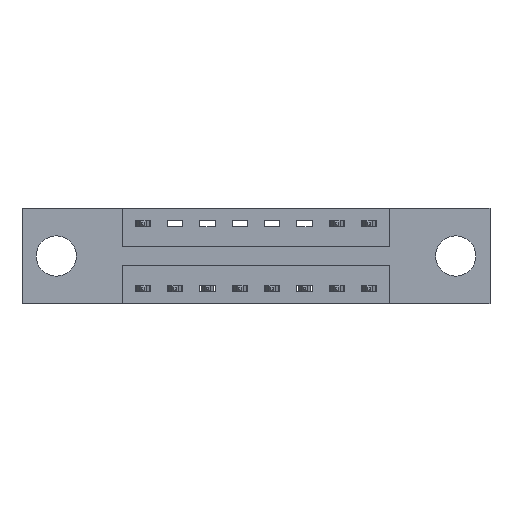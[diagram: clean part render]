
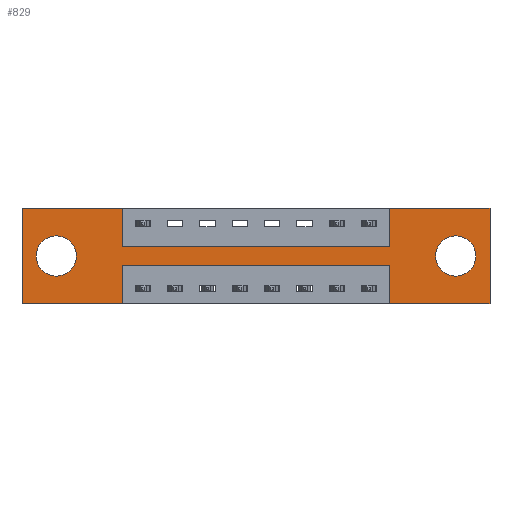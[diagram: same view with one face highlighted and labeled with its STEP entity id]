
A CAD part, front view. The second image highlights one B-rep face of the part: STEP entity #829.
In plain terms, the highlighted planar face has unit normal (0, -1, 0).
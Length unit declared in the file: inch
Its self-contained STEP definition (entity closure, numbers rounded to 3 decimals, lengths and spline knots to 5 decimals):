
#142 = AXIS2_PLACEMENT_3D ( 'NONE', #3195, #8237, #3962 ) ;
#279 = VERTEX_POINT ( 'NONE', #336 ) ;
#292 = VECTOR ( 'NONE', #1090, 39.37008 ) ;
#336 = CARTESIAN_POINT ( 'NONE',  ( 0.1325, 0., -0.107 ) ) ;
#423 = ORIENTED_EDGE ( 'NONE', *, *, #8382, .T. ) ;
#425 = ORIENTED_EDGE ( 'NONE', *, *, #6639, .T. ) ;
#449 = ORIENTED_EDGE ( 'NONE', *, *, #6753, .T. ) ;
#463 = ORIENTED_EDGE ( 'NONE', *, *, #4237, .T. ) ;
#499 = ORIENTED_EDGE ( 'NONE', *, *, #6702, .F. ) ;
#525 = ORIENTED_EDGE ( 'NONE', *, *, #2740, .F. ) ;
#550 = CARTESIAN_POINT ( 'NONE',  ( 0.1325, 0., -0.263 ) ) ;
#573 = VERTEX_POINT ( 'NONE', #4162 ) ;
#583 = EDGE_CURVE ( 'NONE', #5346, #4613, #7836, .T. ) ;
#586 = EDGE_CURVE ( 'NONE', #573, #3477, #4030, .T. ) ;
#593 = ORIENTED_EDGE ( 'NONE', *, *, #5875, .F. ) ;
#601 = VECTOR ( 'NONE', #5198, 39.37008 ) ;
#605 = ORIENTED_EDGE ( 'NONE', *, *, #6371, .F. ) ;
#628 = ORIENTED_EDGE ( 'NONE', *, *, #583, .F. ) ;
#641 = ORIENTED_EDGE ( 'NONE', *, *, #2733, .F. ) ;
#718 = ORIENTED_EDGE ( 'NONE', *, *, #4485, .F. ) ;
#726 = ORIENTED_EDGE ( 'NONE', *, *, #7225, .F. ) ;
#733 = DIRECTION ( 'NONE',  ( -1., 0., 0. ) ) ;
#740 = ORIENTED_EDGE ( 'NONE', *, *, #7984, .F. ) ;
#758 = ORIENTED_EDGE ( 'NONE', *, *, #917, .F. ) ;
#784 = ORIENTED_EDGE ( 'NONE', *, *, #586, .F. ) ;
#799 = ORIENTED_EDGE ( 'NONE', *, *, #5940, .F. ) ;
#829 = ADVANCED_FACE ( 'NONE', ( #8956, #7419, #3541 ), #6366, .T. ) ;
#863 = CARTESIAN_POINT ( 'NONE',  ( 0., 0., -0.37 ) ) ;
#917 = EDGE_CURVE ( 'NONE', #3477, #3834, #6570, .T. ) ;
#1001 = CARTESIAN_POINT ( 'NONE',  ( 0.3875, 0., -0.22 ) ) ;
#1013 = EDGE_LOOP ( 'NONE', ( #499, #525, #593, #605, #628, #641, #718, #726, #740, #758, #784, #799 ) ) ;
#1061 = DIRECTION ( 'NONE',  ( 0., 1., 0. ) ) ;
#1090 = DIRECTION ( 'NONE',  ( 1., 0., 0. ) ) ;
#1217 = CARTESIAN_POINT ( 'NONE',  ( 0., 0., 0. ) ) ;
#1274 = AXIS2_PLACEMENT_3D ( 'NONE', #2845, #7930, #3636 ) ;
#1419 = CARTESIAN_POINT ( 'NONE',  ( 1.81, 0., 0. ) ) ;
#1468 = DIRECTION ( 'NONE',  ( 1., 0., 0. ) ) ;
#1776 = DIRECTION ( 'NONE',  ( 0., 0., -1. ) ) ;
#1845 = CARTESIAN_POINT ( 'NONE',  ( 0.1325, 0., -0.185 ) ) ;
#1919 = VECTOR ( 'NONE', #2865, 39.37008 ) ;
#2191 = DIRECTION ( 'NONE',  ( 0., 0., 1. ) ) ;
#2346 = VERTEX_POINT ( 'NONE', #7579 ) ;
#2568 = VERTEX_POINT ( 'NONE', #4246 ) ;
#2572 = VERTEX_POINT ( 'NONE', #4074 ) ;
#2584 = CIRCLE ( 'NONE', #8445, 0.078 ) ;
#2590 = VERTEX_POINT ( 'NONE', #3718 ) ;
#2674 = DIRECTION ( 'NONE',  ( 0., 0., 1. ) ) ;
#2722 = DIRECTION ( 'NONE',  ( 0., 0., -1. ) ) ;
#2733 = EDGE_CURVE ( 'NONE', #4979, #5346, #4785, .T. ) ;
#2740 = EDGE_CURVE ( 'NONE', #7652, #2568, #6759, .T. ) ;
#2744 = VERTEX_POINT ( 'NONE', #550 ) ;
#2828 = LINE ( 'NONE', #9164, #292 ) ;
#2845 = CARTESIAN_POINT ( 'NONE',  ( 0.1325, 0., -0.185 ) ) ;
#2865 = DIRECTION ( 'NONE',  ( 0., 0., 1. ) ) ;
#2995 = CARTESIAN_POINT ( 'NONE',  ( 1.81, 0., 0. ) ) ;
#3048 = CARTESIAN_POINT ( 'NONE',  ( 0.3875, 0., -0.15 ) ) ;
#3117 = CARTESIAN_POINT ( 'NONE',  ( 1.81, 0., -0.37 ) ) ;
#3195 = CARTESIAN_POINT ( 'NONE',  ( 1.6775, 0., -0.185 ) ) ;
#3384 = CARTESIAN_POINT ( 'NONE',  ( 0.3875, 0., 0. ) ) ;
#3477 = VERTEX_POINT ( 'NONE', #5717 ) ;
#3541 = FACE_OUTER_BOUND ( 'NONE', #1013, .T. ) ;
#3591 = VECTOR ( 'NONE', #2191, 39.37008 ) ;
#3636 = DIRECTION ( 'NONE',  ( 0., 0., 1. ) ) ;
#3718 = CARTESIAN_POINT ( 'NONE',  ( 1.4225, 0., -0.15 ) ) ;
#3834 = VERTEX_POINT ( 'NONE', #5977 ) ;
#3896 = CARTESIAN_POINT ( 'NONE',  ( 0., 0., 0. ) ) ;
#3962 = DIRECTION ( 'NONE',  ( 0., 0., -1. ) ) ;
#4030 = LINE ( 'NONE', #3896, #1919 ) ;
#4052 = LINE ( 'NONE', #863, #6048 ) ;
#4074 = CARTESIAN_POINT ( 'NONE',  ( 1.6775, 0., -0.107 ) ) ;
#4097 = EDGE_LOOP ( 'NONE', ( #449, #463 ) ) ;
#4162 = CARTESIAN_POINT ( 'NONE',  ( 0., 0., -0.37 ) ) ;
#4237 = EDGE_CURVE ( 'NONE', #2744, #279, #6414, .T. ) ;
#4246 = CARTESIAN_POINT ( 'NONE',  ( 0.3875, 0., -0.22 ) ) ;
#4265 = VECTOR ( 'NONE', #2722, 39.37008 ) ;
#4300 = CARTESIAN_POINT ( 'NONE',  ( 0.3875, 0., -0.37 ) ) ;
#4368 = DIRECTION ( 'NONE',  ( 0., -1., 0. ) ) ;
#4375 = CARTESIAN_POINT ( 'NONE',  ( 1.4225, 0., -0.37 ) ) ;
#4378 = CIRCLE ( 'NONE', #142, 0.078 ) ;
#4485 = EDGE_CURVE ( 'NONE', #2590, #4979, #5617, .T. ) ;
#4574 = VECTOR ( 'NONE', #733, 39.37008 ) ;
#4613 = VERTEX_POINT ( 'NONE', #3117 ) ;
#4741 = CARTESIAN_POINT ( 'NONE',  ( 0., 0., 0. ) ) ;
#4785 = LINE ( 'NONE', #1217, #8330 ) ;
#4799 = DIRECTION ( 'NONE',  ( -1., 0., 0. ) ) ;
#4979 = VERTEX_POINT ( 'NONE', #7809 ) ;
#5130 = DIRECTION ( 'NONE',  ( 0., 0., 1. ) ) ;
#5198 = DIRECTION ( 'NONE',  ( -1., 0., 0. ) ) ;
#5225 = DIRECTION ( 'NONE',  ( 0., 0., -1. ) ) ;
#5276 = EDGE_LOOP ( 'NONE', ( #423, #425 ) ) ;
#5295 = CARTESIAN_POINT ( 'NONE',  ( 1.4225, 0., 0. ) ) ;
#5346 = VERTEX_POINT ( 'NONE', #1419 ) ;
#5617 = LINE ( 'NONE', #5295, #3591 ) ;
#5717 = CARTESIAN_POINT ( 'NONE',  ( 0., 0., 0. ) ) ;
#5771 = CARTESIAN_POINT ( 'NONE',  ( 1.6775, 0., -0.185 ) ) ;
#5875 = EDGE_CURVE ( 'NONE', #2346, #7652, #7254, .T. ) ;
#5929 = VECTOR ( 'NONE', #7217, 39.37008 ) ;
#5940 = EDGE_CURVE ( 'NONE', #6202, #573, #6818, .T. ) ;
#5977 = CARTESIAN_POINT ( 'NONE',  ( 0.3875, 0., 0. ) ) ;
#6048 = VECTOR ( 'NONE', #4799, 39.37008 ) ;
#6163 = LINE ( 'NONE', #4300, #5929 ) ;
#6202 = VERTEX_POINT ( 'NONE', #9500 ) ;
#6332 = CARTESIAN_POINT ( 'NONE',  ( 1.6775, 0., -0.263 ) ) ;
#6366 = PLANE ( 'NONE',  #7012 ) ;
#6371 = EDGE_CURVE ( 'NONE', #4613, #2346, #4052, .T. ) ;
#6406 = AXIS2_PLACEMENT_3D ( 'NONE', #1845, #7132, #2674 ) ;
#6414 = CIRCLE ( 'NONE', #6406, 0.078 ) ;
#6503 = DIRECTION ( 'NONE',  ( 0., 0., -1. ) ) ;
#6570 = LINE ( 'NONE', #4741, #8355 ) ;
#6639 = EDGE_CURVE ( 'NONE', #8516, #2572, #2584, .T. ) ;
#6702 = EDGE_CURVE ( 'NONE', #2568, #6202, #6163, .T. ) ;
#6753 = EDGE_CURVE ( 'NONE', #279, #2744, #8381, .T. ) ;
#6759 = LINE ( 'NONE', #1001, #4574 ) ;
#6818 = LINE ( 'NONE', #7312, #601 ) ;
#6930 = CARTESIAN_POINT ( 'NONE',  ( 0., 0., -0.37 ) ) ;
#7012 = AXIS2_PLACEMENT_3D ( 'NONE', #6930, #4368, #5225 ) ;
#7132 = DIRECTION ( 'NONE',  ( 0., 1., 0. ) ) ;
#7217 = DIRECTION ( 'NONE',  ( 0., 0., -1. ) ) ;
#7225 = EDGE_CURVE ( 'NONE', #7510, #2590, #2828, .T. ) ;
#7254 = LINE ( 'NONE', #4375, #8796 ) ;
#7312 = CARTESIAN_POINT ( 'NONE',  ( 0., 0., -0.37 ) ) ;
#7419 = FACE_BOUND ( 'NONE', #4097, .T. ) ;
#7510 = VERTEX_POINT ( 'NONE', #3048 ) ;
#7521 = LINE ( 'NONE', #3384, #9064 ) ;
#7579 = CARTESIAN_POINT ( 'NONE',  ( 1.4225, 0., -0.37 ) ) ;
#7652 = VERTEX_POINT ( 'NONE', #9478 ) ;
#7809 = CARTESIAN_POINT ( 'NONE',  ( 1.4225, 0., 0. ) ) ;
#7836 = LINE ( 'NONE', #2995, #4265 ) ;
#7930 = DIRECTION ( 'NONE',  ( 0., 1., 0. ) ) ;
#7984 = EDGE_CURVE ( 'NONE', #3834, #7510, #7521, .T. ) ;
#8237 = DIRECTION ( 'NONE',  ( 0., 1., 0. ) ) ;
#8330 = VECTOR ( 'NONE', #1468, 39.37008 ) ;
#8355 = VECTOR ( 'NONE', #9390, 39.37008 ) ;
#8381 = CIRCLE ( 'NONE', #1274, 0.078 ) ;
#8382 = EDGE_CURVE ( 'NONE', #2572, #8516, #4378, .T. ) ;
#8445 = AXIS2_PLACEMENT_3D ( 'NONE', #5771, #1061, #6503 ) ;
#8516 = VERTEX_POINT ( 'NONE', #6332 ) ;
#8796 = VECTOR ( 'NONE', #5130, 39.37008 ) ;
#8956 = FACE_BOUND ( 'NONE', #5276, .T. ) ;
#9064 = VECTOR ( 'NONE', #1776, 39.37008 ) ;
#9164 = CARTESIAN_POINT ( 'NONE',  ( 0.3875, 0., -0.15 ) ) ;
#9390 = DIRECTION ( 'NONE',  ( 1., 0., 0. ) ) ;
#9478 = CARTESIAN_POINT ( 'NONE',  ( 1.4225, 0., -0.22 ) ) ;
#9500 = CARTESIAN_POINT ( 'NONE',  ( 0.3875, 0., -0.37 ) ) ;
